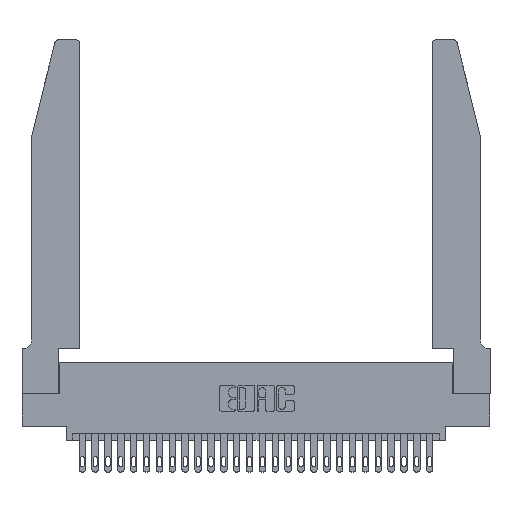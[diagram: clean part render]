
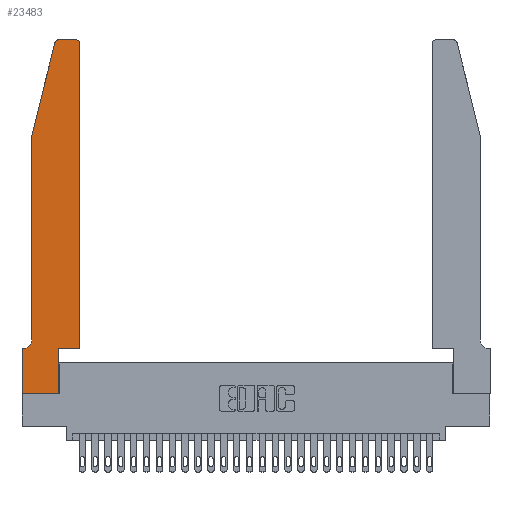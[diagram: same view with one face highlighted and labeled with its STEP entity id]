
A CAD part, top view. The second image highlights one B-rep face of the part: STEP entity #23483.
In plain terms, the highlighted planar face has unit normal (0, 0, 1).
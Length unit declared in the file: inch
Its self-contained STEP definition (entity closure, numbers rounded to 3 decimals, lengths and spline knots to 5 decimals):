
#13 = VERTEX_POINT ( 'NONE', #17834 ) ;
#477 = DIRECTION ( 'NONE',  ( 1., 0., 0. ) ) ;
#625 = CARTESIAN_POINT ( 'NONE',  ( 0.284, 2.72, 0.37 ) ) ;
#866 = VECTOR ( 'NONE', #6058, 39.37008 ) ;
#1296 = EDGE_CURVE ( 'NONE', #19181, #21086, #24110, .T. ) ;
#1544 = VERTEX_POINT ( 'NONE', #13032 ) ;
#1695 = VECTOR ( 'NONE', #13600, 39.37008 ) ;
#1770 = EDGE_CURVE ( 'NONE', #11493, #9540, #7086, .T. ) ;
#1778 = LINE ( 'NONE', #27741, #28449 ) ;
#1789 = DIRECTION ( 'NONE',  ( 0., 1., 0. ) ) ;
#2232 = ORIENTED_EDGE ( 'NONE', *, *, #1296, .T. ) ;
#2462 = EDGE_CURVE ( 'NONE', #13, #23123, #6705, .T. ) ;
#3538 = CARTESIAN_POINT ( 'NONE',  ( 0.4505, 0.35, 0.37 ) ) ;
#4098 = CARTESIAN_POINT ( 'NONE',  ( 0.284, 2.75, 0.37 ) ) ;
#4316 = ORIENTED_EDGE ( 'NONE', *, *, #2462, .T. ) ;
#4328 = DIRECTION ( 'NONE',  ( 0., 0., -1. ) ) ;
#4802 = DIRECTION ( 'NONE',  ( 0., 0., 1. ) ) ;
#4907 = PLANE ( 'NONE',  #21831 ) ;
#5629 = CIRCLE ( 'NONE', #6607, 0.03 ) ;
#6058 = DIRECTION ( 'NONE',  ( 0., -1., 0. ) ) ;
#6395 = VECTOR ( 'NONE', #1789, 39.37008 ) ;
#6598 = VECTOR ( 'NONE', #7708, 39.37008 ) ;
#6607 = AXIS2_PLACEMENT_3D ( 'NONE', #20656, #22578, #7369 ) ;
#6705 = LINE ( 'NONE', #12670, #866 ) ;
#6751 = VECTOR ( 'NONE', #23436, 39.37008 ) ;
#6818 = CARTESIAN_POINT ( 'NONE',  ( 0.0055, 0.42, 0.37 ) ) ;
#7086 = LINE ( 'NONE', #20333, #11286 ) ;
#7369 = DIRECTION ( 'NONE',  ( 1., 0., 0. ) ) ;
#7708 = DIRECTION ( 'NONE',  ( -0.239, -0.971, 0. ) ) ;
#7856 = DIRECTION ( 'NONE',  ( 1., 0., 0. ) ) ;
#7896 = FACE_OUTER_BOUND ( 'NONE', #18471, .T. ) ;
#7973 = CARTESIAN_POINT ( 'NONE',  ( 0.0755, 0.42, 0.37 ) ) ;
#8012 = VERTEX_POINT ( 'NONE', #3538 ) ;
#8152 = ORIENTED_EDGE ( 'NONE', *, *, #8257, .T. ) ;
#8241 = EDGE_CURVE ( 'NONE', #11526, #16144, #9060, .T. ) ;
#8257 = EDGE_CURVE ( 'NONE', #1544, #13, #17366, .T. ) ;
#8469 = EDGE_CURVE ( 'NONE', #8012, #13789, #1778, .T. ) ;
#8795 = CIRCLE ( 'NONE', #14428, 0.03 ) ;
#9060 = LINE ( 'NONE', #24073, #14293 ) ;
#9079 = DIRECTION ( 'NONE',  ( -1., 0., 0. ) ) ;
#9102 = ORIENTED_EDGE ( 'NONE', *, *, #16724, .T. ) ;
#9342 = CARTESIAN_POINT ( 'NONE',  ( 0., 0., 0.37 ) ) ;
#9451 = VERTEX_POINT ( 'NONE', #13487 ) ;
#9540 = VERTEX_POINT ( 'NONE', #27491 ) ;
#10045 = CARTESIAN_POINT ( 'NONE',  ( 0.2865, 0.35, 0.37 ) ) ;
#11286 = VECTOR ( 'NONE', #7856, 39.37008 ) ;
#11493 = VERTEX_POINT ( 'NONE', #9342 ) ;
#11526 = VERTEX_POINT ( 'NONE', #11777 ) ;
#11676 = EDGE_CURVE ( 'NONE', #9540, #9451, #20982, .T. ) ;
#11710 = AXIS2_PLACEMENT_3D ( 'NONE', #6818, #4328, #9079 ) ;
#11777 = CARTESIAN_POINT ( 'NONE',  ( 0.0055, 0.35, 0.37 ) ) ;
#12251 = ORIENTED_EDGE ( 'NONE', *, *, #27647, .T. ) ;
#12566 = EDGE_CURVE ( 'NONE', #21086, #1544, #8795, .T. ) ;
#12567 = CARTESIAN_POINT ( 'NONE',  ( 0.0755, 2., 0.37 ) ) ;
#12670 = CARTESIAN_POINT ( 'NONE',  ( 0.0755, 2., 0.37 ) ) ;
#13032 = CARTESIAN_POINT ( 'NONE',  ( 0.25487, 2.72718, 0.37 ) ) ;
#13036 = ORIENTED_EDGE ( 'NONE', *, *, #11676, .T. ) ;
#13098 = ORIENTED_EDGE ( 'NONE', *, *, #8241, .T. ) ;
#13370 = EDGE_CURVE ( 'NONE', #13789, #19181, #5629, .T. ) ;
#13487 = CARTESIAN_POINT ( 'NONE',  ( 0.2865, 0.35, 0.37 ) ) ;
#13600 = DIRECTION ( 'NONE',  ( 0., -1., 0. ) ) ;
#13789 = VERTEX_POINT ( 'NONE', #15513 ) ;
#14195 = DIRECTION ( 'NONE',  ( 0., 0., 1. ) ) ;
#14226 = ORIENTED_EDGE ( 'NONE', *, *, #13370, .T. ) ;
#14293 = VECTOR ( 'NONE', #17416, 39.37008 ) ;
#14428 = AXIS2_PLACEMENT_3D ( 'NONE', #625, #14195, #25321 ) ;
#14583 = CIRCLE ( 'NONE', #11710, 0.07 ) ;
#15153 = ORIENTED_EDGE ( 'NONE', *, *, #8469, .T. ) ;
#15268 = ORIENTED_EDGE ( 'NONE', *, *, #1770, .T. ) ;
#15513 = CARTESIAN_POINT ( 'NONE',  ( 0.4505, 2.72, 0.37 ) ) ;
#16144 = VERTEX_POINT ( 'NONE', #25748 ) ;
#16724 = EDGE_CURVE ( 'NONE', #9451, #8012, #23569, .T. ) ;
#16741 = CARTESIAN_POINT ( 'NONE',  ( 0.4505, 0.35, 0.37 ) ) ;
#17366 = LINE ( 'NONE', #12567, #6598 ) ;
#17416 = DIRECTION ( 'NONE',  ( -1., 0., 0. ) ) ;
#17601 = ORIENTED_EDGE ( 'NONE', *, *, #25196, .T. ) ;
#17834 = CARTESIAN_POINT ( 'NONE',  ( 0.0755, 2., 0.37 ) ) ;
#18189 = CARTESIAN_POINT ( 'NONE',  ( 0., 0.35, 0.37 ) ) ;
#18252 = CARTESIAN_POINT ( 'NONE',  ( 0., 0., 0.37 ) ) ;
#18471 = EDGE_LOOP ( 'NONE', ( #2232, #22443, #8152, #4316, #17601, #13098, #12251, #15268, #13036, #9102, #15153, #14226 ) ) ;
#18810 = CARTESIAN_POINT ( 'NONE',  ( 0.2605, 2.75, 0.37 ) ) ;
#19181 = VERTEX_POINT ( 'NONE', #25036 ) ;
#20333 = CARTESIAN_POINT ( 'NONE',  ( 0., 0., 0.37 ) ) ;
#20656 = CARTESIAN_POINT ( 'NONE',  ( 0.4205, 2.72, 0.37 ) ) ;
#20982 = LINE ( 'NONE', #10045, #6395 ) ;
#21086 = VERTEX_POINT ( 'NONE', #4098 ) ;
#21251 = DIRECTION ( 'NONE',  ( 0., 1., 0. ) ) ;
#21502 = VECTOR ( 'NONE', #25608, 39.37008 ) ;
#21831 = AXIS2_PLACEMENT_3D ( 'NONE', #18189, #4802, #477 ) ;
#22443 = ORIENTED_EDGE ( 'NONE', *, *, #12566, .T. ) ;
#22578 = DIRECTION ( 'NONE',  ( 0., 0., 1. ) ) ;
#23123 = VERTEX_POINT ( 'NONE', #7973 ) ;
#23436 = DIRECTION ( 'NONE',  ( -1., 0., 0. ) ) ;
#23483 = ADVANCED_FACE ( 'NONE', ( #7896 ), #4907, .T. ) ;
#23569 = LINE ( 'NONE', #16741, #21502 ) ;
#24073 = CARTESIAN_POINT ( 'NONE',  ( 0.0755, 0.35, 0.37 ) ) ;
#24110 = LINE ( 'NONE', #18810, #6751 ) ;
#25036 = CARTESIAN_POINT ( 'NONE',  ( 0.4205, 2.75, 0.37 ) ) ;
#25196 = EDGE_CURVE ( 'NONE', #23123, #11526, #14583, .T. ) ;
#25321 = DIRECTION ( 'NONE',  ( 1., 0., 0. ) ) ;
#25608 = DIRECTION ( 'NONE',  ( 1., 0., 0. ) ) ;
#25748 = CARTESIAN_POINT ( 'NONE',  ( 0., 0.35, 0.37 ) ) ;
#26298 = LINE ( 'NONE', #18252, #1695 ) ;
#27491 = CARTESIAN_POINT ( 'NONE',  ( 0.2865, 0., 0.37 ) ) ;
#27647 = EDGE_CURVE ( 'NONE', #16144, #11493, #26298, .T. ) ;
#27741 = CARTESIAN_POINT ( 'NONE',  ( 0.4505, 0.35, 0.37 ) ) ;
#28449 = VECTOR ( 'NONE', #21251, 39.37008 ) ;
